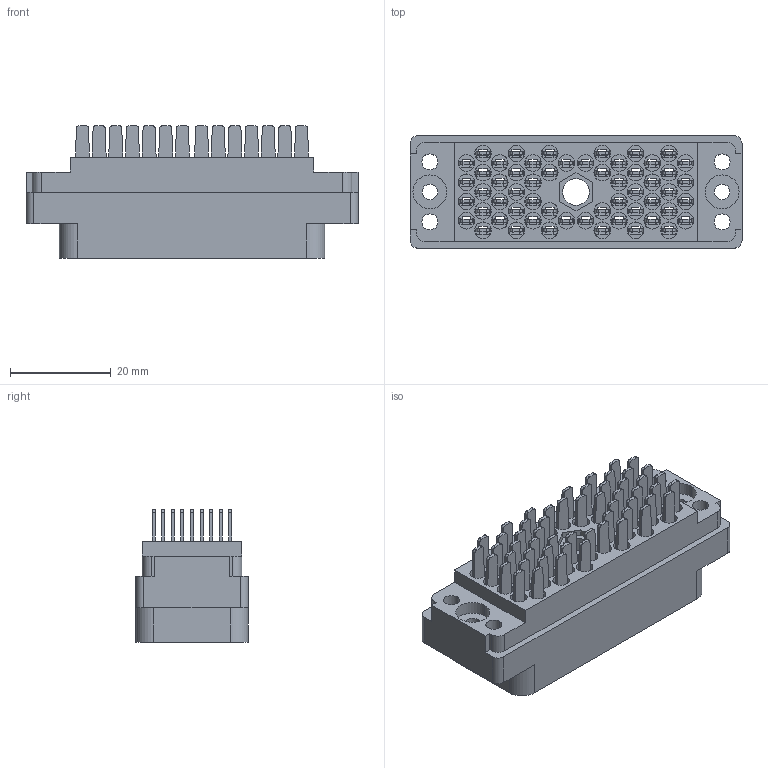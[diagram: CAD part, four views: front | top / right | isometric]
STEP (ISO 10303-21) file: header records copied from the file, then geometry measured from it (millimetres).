
FILE_DESCRIPTION (( 'STEP AP203' ), '1' );
FILE_NAME ('516-056-501-300.STEP', '2020-09-08T05:05:34', ( '' ), ( '' ), 'SwSTEP 2.0', 'SolidWorks 2020', '' );
FILE_SCHEMA (( 'CONFIG_CONTROL_DESIGN' ));
Length unit declared in the file: inch
Products named in the file (3): 516-292-001_501 Contact; 516 Plug Insulator_056; 516-056-501-300
Assembly tree (57 placements, depth 2):
  516-056-501-300
    516 Plug Insulator_056
    516-292-001_501 Contact  x56
Bounding box: 65.81 x 22.25 x 26.26 mm (x, y, z)
Volume: 13456.5 mm3; surface area: 25713.8 mm2
Topology: 57 solids, 57 shells, 5250 faces, 15244 edges, 10124 vertices
Faces by surface type: plane 3193, cylinder 1719, bspline 336, cone 2
Entity records: 45482 total; most frequent: CARTESIAN_POINT 7973, ORIENTED_EDGE 7608, DIRECTION 7362, EDGE_CURVE 3804, VECTOR 2866, LINE 2866, VERTEX_POINT 2534, AXIS2_PLACEMENT_3D 2248
